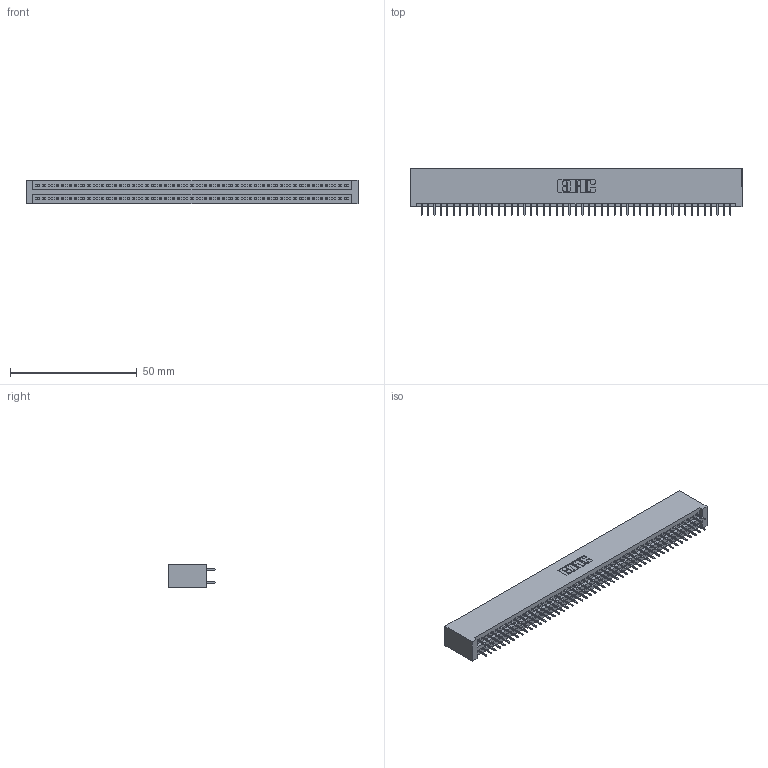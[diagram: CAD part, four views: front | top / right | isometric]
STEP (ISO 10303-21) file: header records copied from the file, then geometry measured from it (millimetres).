
FILE_DESCRIPTION (( 'STEP AP203' ), '1' );
FILE_NAME ('395-098-525-201.STEP', '2020-09-25T15:28:59', ( '' ), ( '' ), 'SwSTEP 2.0', 'SolidWorks 2020', '' );
FILE_SCHEMA (( 'CONFIG_CONTROL_DESIGN' ));
Length unit declared in the file: inch
Products named in the file (3): 345-292-001_345-293-125; 395-098-525-201; 345 Part_No Mounting Lugs
Assembly tree (99 placements, depth 2):
  395-098-525-201
    345 Part_No Mounting Lugs
    345-292-001_345-293-125  x98
Bounding box: 131.06 x 18.72 x 9.4 mm (x, y, z)
Volume: 13251.3 mm3; surface area: 19540.4 mm2
Topology: 99 solids, 99 shells, 5410 faces, 15311 edges, 9814 vertices
Faces by surface type: plane 3898, cylinder 1512
Entity records: 37301 total; most frequent: CARTESIAN_POINT 6244, ORIENTED_EDGE 6178, DIRECTION 5493, EDGE_CURVE 3089, LINE 2773, VECTOR 2773, VERTEX_POINT 2054, AXIS2_PLACEMENT_3D 1360
